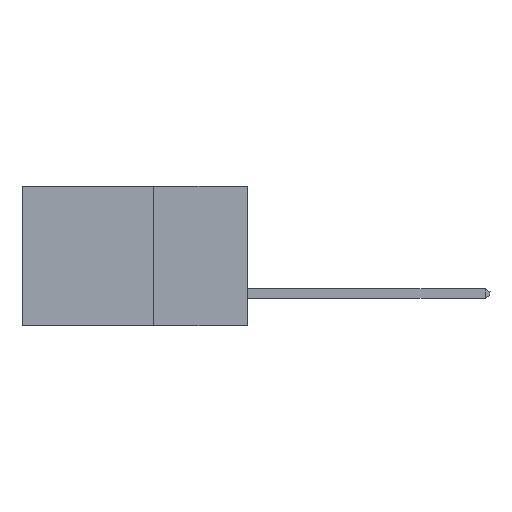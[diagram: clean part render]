
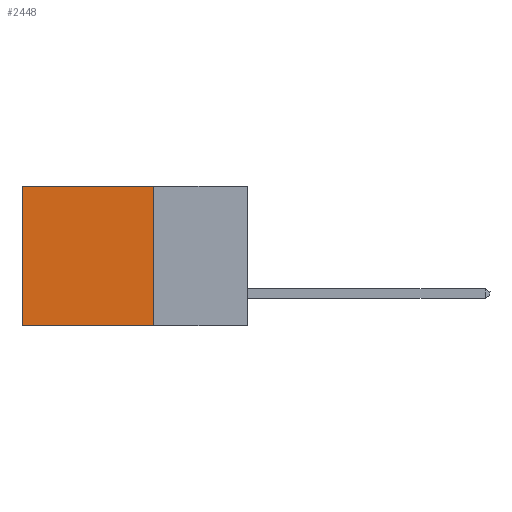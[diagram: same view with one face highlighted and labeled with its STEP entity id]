
A CAD part, left-side view. The second image highlights one B-rep face of the part: STEP entity #2448.
In plain terms, the highlighted planar face has unit normal (-1, 0, 0).
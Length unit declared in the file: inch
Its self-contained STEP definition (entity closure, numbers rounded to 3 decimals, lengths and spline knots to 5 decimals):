
#775 = VECTOR ( 'NONE', #5444, 39.37008 ) ;
#1080 = VERTEX_POINT ( 'NONE', #2565 ) ;
#1093 = DIRECTION ( 'NONE',  ( 0., 1., 0. ) ) ;
#1525 = ORIENTED_EDGE ( 'NONE', *, *, #4753, .T. ) ;
#2032 = VERTEX_POINT ( 'NONE', #6260 ) ;
#2448 = ADVANCED_FACE ( 'NONE', ( #5608 ), #5433, .F. ) ;
#2565 = CARTESIAN_POINT ( 'NONE',  ( 0.2615, 0.6, -0.37 ) ) ;
#2988 = VECTOR ( 'NONE', #1093, 39.37008 ) ;
#3027 = LINE ( 'NONE', #8426, #6734 ) ;
#3625 = CARTESIAN_POINT ( 'NONE',  ( 0.2615, 0.25, -0.37 ) ) ;
#3819 = LINE ( 'NONE', #11025, #2988 ) ;
#3845 = DIRECTION ( 'NONE',  ( 1., 0., 0. ) ) ;
#4060 = CARTESIAN_POINT ( 'NONE',  ( 0.2615, 0.25, 0. ) ) ;
#4410 = DIRECTION ( 'NONE',  ( 0., 1., 0. ) ) ;
#4753 = EDGE_CURVE ( 'NONE', #10767, #2032, #8705, .T. ) ;
#5358 = ORIENTED_EDGE ( 'NONE', *, *, #7882, .T. ) ;
#5433 = PLANE ( 'NONE',  #6287 ) ;
#5444 = DIRECTION ( 'NONE',  ( 0., 0., -1. ) ) ;
#5582 = ORIENTED_EDGE ( 'NONE', *, *, #8292, .F. ) ;
#5608 = FACE_OUTER_BOUND ( 'NONE', #6752, .T. ) ;
#5758 = DIRECTION ( 'NONE',  ( 0., 0., -1. ) ) ;
#6260 = CARTESIAN_POINT ( 'NONE',  ( 0.2615, 0.6, 0. ) ) ;
#6287 = AXIS2_PLACEMENT_3D ( 'NONE', #9133, #3845, #10868 ) ;
#6734 = VECTOR ( 'NONE', #5758, 39.37008 ) ;
#6752 = EDGE_LOOP ( 'NONE', ( #5358, #5582, #8046, #1525 ) ) ;
#7097 = VECTOR ( 'NONE', #4410, 39.37008 ) ;
#7503 = EDGE_CURVE ( 'NONE', #10767, #10522, #10940, .T. ) ;
#7882 = EDGE_CURVE ( 'NONE', #2032, #1080, #3027, .T. ) ;
#8046 = ORIENTED_EDGE ( 'NONE', *, *, #7503, .F. ) ;
#8292 = EDGE_CURVE ( 'NONE', #10522, #1080, #3819, .T. ) ;
#8426 = CARTESIAN_POINT ( 'NONE',  ( 0.2615, 0.6, -0.37 ) ) ;
#8705 = LINE ( 'NONE', #9741, #7097 ) ;
#9133 = CARTESIAN_POINT ( 'NONE',  ( 0.2615, 0.25, -0.37 ) ) ;
#9741 = CARTESIAN_POINT ( 'NONE',  ( 0.2615, 0.25, 0. ) ) ;
#10173 = CARTESIAN_POINT ( 'NONE',  ( 0.2615, 0.25, -0.37 ) ) ;
#10522 = VERTEX_POINT ( 'NONE', #10173 ) ;
#10767 = VERTEX_POINT ( 'NONE', #4060 ) ;
#10868 = DIRECTION ( 'NONE',  ( 0., 0., -1. ) ) ;
#10940 = LINE ( 'NONE', #3625, #775 ) ;
#11025 = CARTESIAN_POINT ( 'NONE',  ( 0.2615, 0.25, -0.37 ) ) ;
